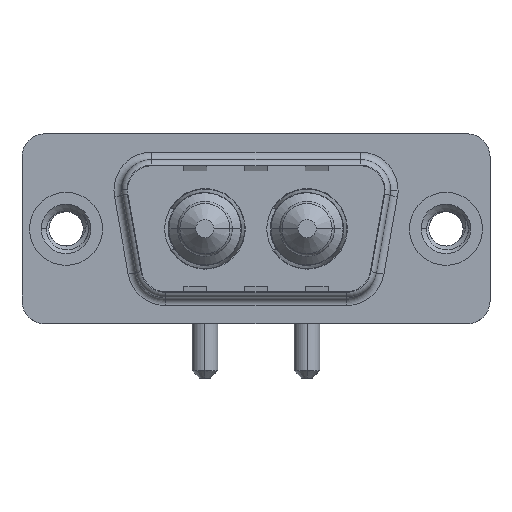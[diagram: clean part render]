
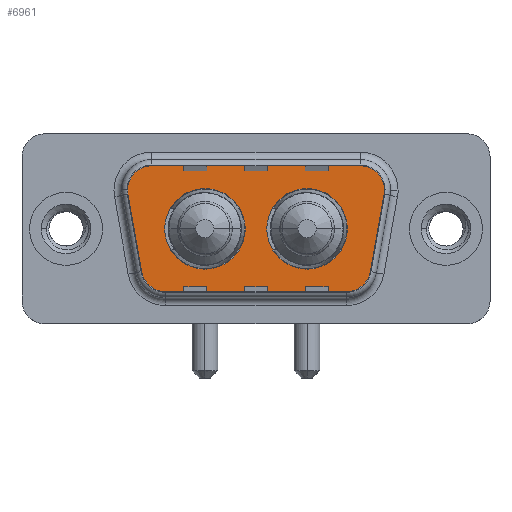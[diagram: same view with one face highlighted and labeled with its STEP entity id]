
A CAD part, top view. The second image highlights one B-rep face of the part: STEP entity #6961.
In plain terms, the highlighted planar face has unit normal (0, 0, 1).
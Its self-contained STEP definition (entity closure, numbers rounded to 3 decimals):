
#41 = EDGE_CURVE ( 'NONE', #7071, #9273, #449, .T. ) ;
#69 = DIRECTION ( 'NONE',  ( 0., 0., 1. ) ) ;
#81 = CARTESIAN_POINT ( 'NONE',  ( 9.14, 0., 0. ) ) ;
#174 = FACE_BOUND ( 'NONE', #2327, .T. ) ;
#449 = CIRCLE ( 'NONE', #1945, 2.65 ) ;
#678 = CIRCLE ( 'NONE', #2179, 2.65 ) ;
#770 = EDGE_CURVE ( 'NONE', #8279, #3004, #9640, .T. ) ;
#838 = DIRECTION ( 'NONE',  ( 1., 0., 0. ) ) ;
#867 = EDGE_CURVE ( 'NONE', #3727, #5728, #4356, .T. ) ;
#963 = CARTESIAN_POINT ( 'NONE',  ( 4.489, -3.247, 0. ) ) ;
#1113 = ORIENTED_EDGE ( 'NONE', *, *, #41, .F. ) ;
#1644 = AXIS2_PLACEMENT_3D ( 'NONE', #4991, #8569, #2468 ) ;
#1725 = EDGE_CURVE ( 'NONE', #2716, #8279, #5606, .T. ) ;
#1847 = DIRECTION ( 'NONE',  ( 0., 0., 1. ) ) ;
#1945 = AXIS2_PLACEMENT_3D ( 'NONE', #7899, #10815, #4384 ) ;
#1948 = DIRECTION ( 'NONE',  ( -1., 0., 0. ) ) ;
#2179 = AXIS2_PLACEMENT_3D ( 'NONE', #6318, #10711, #4502 ) ;
#2215 = VERTEX_POINT ( 'NONE', #6220 ) ;
#2327 = EDGE_LOOP ( 'NONE', ( #1113, #4141 ) ) ;
#2417 = EDGE_CURVE ( 'NONE', #3004, #3221, #7858, .T. ) ;
#2467 = VERTEX_POINT ( 'NONE', #3986 ) ;
#2468 = DIRECTION ( 'NONE',  ( -1., 0., 0. ) ) ;
#2473 = DIRECTION ( 'NONE',  ( 0.174, 0.985, 0. ) ) ;
#2482 = DIRECTION ( 'NONE',  ( 0., 0., 1. ) ) ;
#2527 = ORIENTED_EDGE ( 'NONE', *, *, #2417, .T. ) ;
#2544 = AXIS2_PLACEMENT_3D ( 'NONE', #7617, #8385, #6684 ) ;
#2597 = VECTOR ( 'NONE', #1948, 1000. ) ;
#2695 = VERTEX_POINT ( 'NONE', #10601 ) ;
#2716 = VERTEX_POINT ( 'NONE', #6265 ) ;
#2745 = EDGE_CURVE ( 'NONE', #2215, #2467, #678, .T. ) ;
#2814 = PLANE ( 'NONE',  #9778 ) ;
#3004 = VERTEX_POINT ( 'NONE', #963 ) ;
#3126 = CIRCLE ( 'NONE', #11548, 2.65 ) ;
#3221 = VERTEX_POINT ( 'NONE', #10121 ) ;
#3250 = ORIENTED_EDGE ( 'NONE', *, *, #770, .T. ) ;
#3349 = ORIENTED_EDGE ( 'NONE', *, *, #867, .T. ) ;
#3482 = CARTESIAN_POINT ( 'NONE',  ( 21.564, 2.9, 0. ) ) ;
#3651 = LINE ( 'NONE', #9995, #2597 ) ;
#3727 = VERTEX_POINT ( 'NONE', #7719 ) ;
#3781 = EDGE_CURVE ( 'NONE', #5728, #8622, #9622, .T. ) ;
#3792 = CIRCLE ( 'NONE', #10717, 2. ) ;
#3986 = CARTESIAN_POINT ( 'NONE',  ( 6.49, 0., 0. ) ) ;
#4078 = CARTESIAN_POINT ( 'NONE',  ( 19.564, 2.9, 0. ) ) ;
#4141 = ORIENTED_EDGE ( 'NONE', *, *, #10048, .F. ) ;
#4171 = VECTOR ( 'NONE', #8935, 1000. ) ;
#4201 = CARTESIAN_POINT ( 'NONE',  ( 6.459, -4.9, 0. ) ) ;
#4356 = LINE ( 'NONE', #5296, #9055 ) ;
#4358 = CARTESIAN_POINT ( 'NONE',  ( 19.564, 4.9, 0. ) ) ;
#4384 = DIRECTION ( 'NONE',  ( 1., 0., 0. ) ) ;
#4502 = DIRECTION ( 'NONE',  ( 1., 0., 0. ) ) ;
#4801 = ORIENTED_EDGE ( 'NONE', *, *, #3781, .T. ) ;
#4991 = CARTESIAN_POINT ( 'NONE',  ( 19.564, 2.9, 0. ) ) ;
#5193 = DIRECTION ( 'NONE',  ( 0., 0., 1. ) ) ;
#5207 = CARTESIAN_POINT ( 'NONE',  ( 21.534, 2.553, 0. ) ) ;
#5281 = EDGE_CURVE ( 'NONE', #8622, #10476, #9338, .T. ) ;
#5296 = CARTESIAN_POINT ( 'NONE',  ( 21.534, 2.553, 0. ) ) ;
#5606 = CIRCLE ( 'NONE', #6909, 2. ) ;
#5728 = VERTEX_POINT ( 'NONE', #5207 ) ;
#5764 = EDGE_CURVE ( 'NONE', #3221, #2695, #8845, .T. ) ;
#5820 = CARTESIAN_POINT ( 'NONE',  ( 3.466, 2.553, 0. ) ) ;
#5874 = EDGE_CURVE ( 'NONE', #2467, #2215, #11375, .T. ) ;
#5921 = ORIENTED_EDGE ( 'NONE', *, *, #1725, .T. ) ;
#6018 = DIRECTION ( 'NONE',  ( 0., 0., 1. ) ) ;
#6072 = CARTESIAN_POINT ( 'NONE',  ( 5.436, 2.9, 0. ) ) ;
#6220 = CARTESIAN_POINT ( 'NONE',  ( 11.79, 0., 0. ) ) ;
#6265 = CARTESIAN_POINT ( 'NONE',  ( 5.436, 4.9, 0. ) ) ;
#6318 = CARTESIAN_POINT ( 'NONE',  ( 9.14, 0., 0. ) ) ;
#6336 = VECTOR ( 'NONE', #7083, 1000. ) ;
#6394 = EDGE_CURVE ( 'NONE', #10476, #2716, #3651, .T. ) ;
#6462 = DIRECTION ( 'NONE',  ( 1., 0., 0. ) ) ;
#6538 = DIRECTION ( 'NONE',  ( 1., 0., 0. ) ) ;
#6684 = DIRECTION ( 'NONE',  ( -1., 0., 0. ) ) ;
#6885 = CARTESIAN_POINT ( 'NONE',  ( 18.51, 0., 0. ) ) ;
#6909 = AXIS2_PLACEMENT_3D ( 'NONE', #6072, #5193, #6462 ) ;
#6942 = DIRECTION ( 'NONE',  ( 0., 0., 1. ) ) ;
#6944 = DIRECTION ( 'NONE',  ( 1., 0., 0. ) ) ;
#6961 = ADVANCED_FACE ( 'NONE', ( #174, #9980, #10849 ), #2814, .T. ) ;
#7025 = ORIENTED_EDGE ( 'NONE', *, *, #2745, .F. ) ;
#7071 = VERTEX_POINT ( 'NONE', #6885 ) ;
#7083 = DIRECTION ( 'NONE',  ( 1., 0., 0. ) ) ;
#7244 = ORIENTED_EDGE ( 'NONE', *, *, #5874, .F. ) ;
#7384 = ORIENTED_EDGE ( 'NONE', *, *, #7802, .T. ) ;
#7617 = CARTESIAN_POINT ( 'NONE',  ( 6.459, -2.9, 0. ) ) ;
#7719 = CARTESIAN_POINT ( 'NONE',  ( 20.511, -3.247, 0. ) ) ;
#7802 = EDGE_CURVE ( 'NONE', #2695, #3727, #3792, .T. ) ;
#7858 = CIRCLE ( 'NONE', #2544, 2. ) ;
#7899 = CARTESIAN_POINT ( 'NONE',  ( 15.86, 0., 0. ) ) ;
#7958 = ORIENTED_EDGE ( 'NONE', *, *, #5764, .T. ) ;
#8073 = DIRECTION ( 'NONE',  ( 1., 0., 0. ) ) ;
#8090 = EDGE_LOOP ( 'NONE', ( #7384, #3349, #4801, #8996, #10644, #5921, #3250, #2527, #7958 ) ) ;
#8279 = VERTEX_POINT ( 'NONE', #5820 ) ;
#8385 = DIRECTION ( 'NONE',  ( 0., 0., 1. ) ) ;
#8569 = DIRECTION ( 'NONE',  ( 0., 0., 1. ) ) ;
#8622 = VERTEX_POINT ( 'NONE', #3482 ) ;
#8818 = CARTESIAN_POINT ( 'NONE',  ( 3.466, 2.553, 0. ) ) ;
#8845 = LINE ( 'NONE', #4201, #6336 ) ;
#8935 = DIRECTION ( 'NONE',  ( 0.174, -0.985, 0. ) ) ;
#8996 = ORIENTED_EDGE ( 'NONE', *, *, #5281, .T. ) ;
#9055 = VECTOR ( 'NONE', #2473, 1000. ) ;
#9273 = VERTEX_POINT ( 'NONE', #11073 ) ;
#9338 = CIRCLE ( 'NONE', #1644, 2. ) ;
#9585 = CARTESIAN_POINT ( 'NONE',  ( 18.541, -2.9, 0. ) ) ;
#9600 = DIRECTION ( 'NONE',  ( -1., 0., 0. ) ) ;
#9622 = CIRCLE ( 'NONE', #11104, 2. ) ;
#9640 = LINE ( 'NONE', #8818, #4171 ) ;
#9720 = AXIS2_PLACEMENT_3D ( 'NONE', #81, #1847, #8073 ) ;
#9778 = AXIS2_PLACEMENT_3D ( 'NONE', #10518, #2482, #6944 ) ;
#9980 = FACE_BOUND ( 'NONE', #10204, .T. ) ;
#9995 = CARTESIAN_POINT ( 'NONE',  ( 5.436, 4.9, 0. ) ) ;
#10048 = EDGE_CURVE ( 'NONE', #9273, #7071, #3126, .T. ) ;
#10121 = CARTESIAN_POINT ( 'NONE',  ( 6.459, -4.9, 0. ) ) ;
#10204 = EDGE_LOOP ( 'NONE', ( #7025, #7244 ) ) ;
#10476 = VERTEX_POINT ( 'NONE', #4358 ) ;
#10518 = CARTESIAN_POINT ( 'NONE',  ( 18.541, -2.9, 0. ) ) ;
#10601 = CARTESIAN_POINT ( 'NONE',  ( 18.541, -4.9, 0. ) ) ;
#10644 = ORIENTED_EDGE ( 'NONE', *, *, #6394, .T. ) ;
#10711 = DIRECTION ( 'NONE',  ( 0., 0., 1. ) ) ;
#10717 = AXIS2_PLACEMENT_3D ( 'NONE', #9585, #6942, #838 ) ;
#10815 = DIRECTION ( 'NONE',  ( 0., 0., 1. ) ) ;
#10849 = FACE_OUTER_BOUND ( 'NONE', #8090, .T. ) ;
#10925 = CARTESIAN_POINT ( 'NONE',  ( 15.86, 0., 0. ) ) ;
#11073 = CARTESIAN_POINT ( 'NONE',  ( 13.21, 0., 0. ) ) ;
#11104 = AXIS2_PLACEMENT_3D ( 'NONE', #4078, #6018, #9600 ) ;
#11375 = CIRCLE ( 'NONE', #9720, 2.65 ) ;
#11548 = AXIS2_PLACEMENT_3D ( 'NONE', #10925, #69, #6538 ) ;
